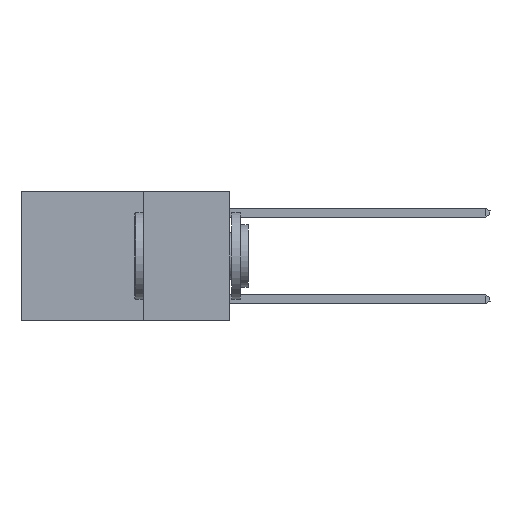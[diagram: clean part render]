
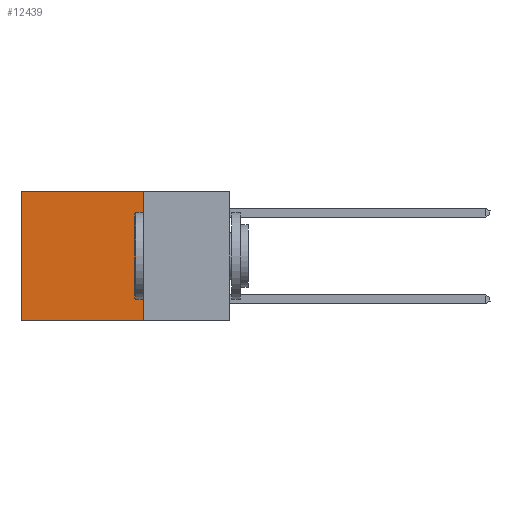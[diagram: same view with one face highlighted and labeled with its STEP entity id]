
A CAD part, left-side view. The second image highlights one B-rep face of the part: STEP entity #12439.
In plain terms, the highlighted planar face has unit normal (-1, 0, 0).
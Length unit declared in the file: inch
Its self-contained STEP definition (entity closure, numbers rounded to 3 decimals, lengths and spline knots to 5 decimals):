
#1791 = EDGE_CURVE ( 'NONE', #5123, #27274, #17716, .T. ) ;
#2206 = CARTESIAN_POINT ( 'NONE',  ( 0.2625, 0.25, 0. ) ) ;
#2275 = LINE ( 'NONE', #18849, #24766 ) ;
#3954 = DIRECTION ( 'NONE',  ( 1., 0., 0. ) ) ;
#4395 = LINE ( 'NONE', #8833, #13134 ) ;
#4549 = EDGE_CURVE ( 'NONE', #9222, #8467, #11884, .T. ) ;
#5089 = EDGE_LOOP ( 'NONE', ( #18928, #18643, #9081, #6774 ) ) ;
#5123 = VERTEX_POINT ( 'NONE', #8650 ) ;
#6237 = FACE_OUTER_BOUND ( 'NONE', #5089, .T. ) ;
#6774 = ORIENTED_EDGE ( 'NONE', *, *, #15425, .T. ) ;
#8467 = VERTEX_POINT ( 'NONE', #15086 ) ;
#8540 = PLANE ( 'NONE',  #15282 ) ;
#8650 = CARTESIAN_POINT ( 'NONE',  ( 0.2625, 0.6, 0. ) ) ;
#8833 = CARTESIAN_POINT ( 'NONE',  ( 0.2625, 0.25, 0. ) ) ;
#9081 = ORIENTED_EDGE ( 'NONE', *, *, #4549, .F. ) ;
#9222 = VERTEX_POINT ( 'NONE', #26937 ) ;
#9473 = VECTOR ( 'NONE', #18012, 39.37008 ) ;
#11884 = LINE ( 'NONE', #27646, #25107 ) ;
#12439 = ADVANCED_FACE ( 'NONE', ( #6237 ), #8540, .F. ) ;
#13134 = VECTOR ( 'NONE', #21969, 39.37008 ) ;
#15086 = CARTESIAN_POINT ( 'NONE',  ( 0.2625, 0.25, -0.37 ) ) ;
#15196 = CARTESIAN_POINT ( 'NONE',  ( 0.2625, 0.6, -0.37 ) ) ;
#15282 = AXIS2_PLACEMENT_3D ( 'NONE', #2206, #3954, #19179 ) ;
#15425 = EDGE_CURVE ( 'NONE', #9222, #5123, #4395, .T. ) ;
#17716 = LINE ( 'NONE', #26617, #9473 ) ;
#18012 = DIRECTION ( 'NONE',  ( 0., 0., -1. ) ) ;
#18509 = EDGE_CURVE ( 'NONE', #8467, #27274, #2275, .T. ) ;
#18643 = ORIENTED_EDGE ( 'NONE', *, *, #18509, .F. ) ;
#18849 = CARTESIAN_POINT ( 'NONE',  ( 0.2625, 0.25, -0.37 ) ) ;
#18928 = ORIENTED_EDGE ( 'NONE', *, *, #1791, .T. ) ;
#19179 = DIRECTION ( 'NONE',  ( 0., 0., -1. ) ) ;
#20662 = DIRECTION ( 'NONE',  ( 0., 0., -1. ) ) ;
#21969 = DIRECTION ( 'NONE',  ( 0., 1., 0. ) ) ;
#22022 = DIRECTION ( 'NONE',  ( 0., 1., 0. ) ) ;
#24766 = VECTOR ( 'NONE', #22022, 39.37008 ) ;
#25107 = VECTOR ( 'NONE', #20662, 39.37008 ) ;
#26617 = CARTESIAN_POINT ( 'NONE',  ( 0.2625, 0.6, 0. ) ) ;
#26937 = CARTESIAN_POINT ( 'NONE',  ( 0.2625, 0.25, 0. ) ) ;
#27274 = VERTEX_POINT ( 'NONE', #15196 ) ;
#27646 = CARTESIAN_POINT ( 'NONE',  ( 0.2625, 0.25, 0. ) ) ;
